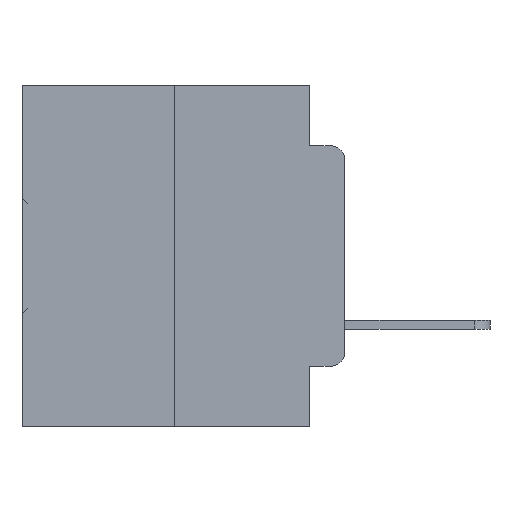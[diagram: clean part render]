
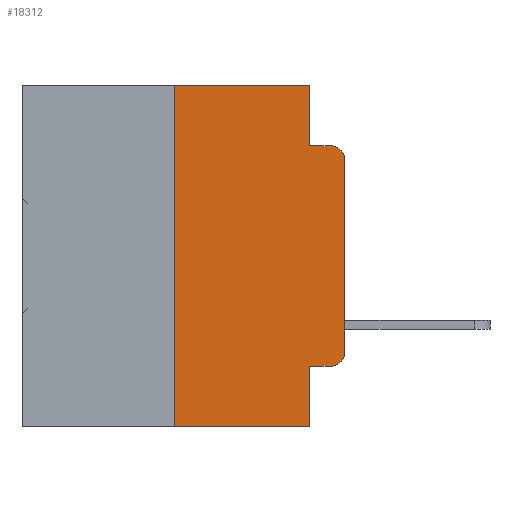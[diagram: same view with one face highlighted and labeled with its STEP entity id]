
A CAD part, left-side view. The second image highlights one B-rep face of the part: STEP entity #18312.
In plain terms, the highlighted planar face has unit normal (-1, 0, 0).
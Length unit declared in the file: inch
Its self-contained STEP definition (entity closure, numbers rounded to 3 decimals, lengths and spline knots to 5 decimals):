
#837 = VECTOR ( 'NONE', #34063, 39.37008 ) ;
#1069 = VERTEX_POINT ( 'NONE', #4931 ) ;
#1289 = DIRECTION ( 'NONE',  ( -1., 0., 0. ) ) ;
#1640 = EDGE_CURVE ( 'NONE', #7655, #21666, #33409, .T. ) ;
#1653 = CARTESIAN_POINT ( 'NONE',  ( 0., 0.051, -0.5 ) ) ;
#2435 = CARTESIAN_POINT ( 'NONE',  ( 0., 0.25, 0. ) ) ;
#2543 = DIRECTION ( 'NONE',  ( 0., 0., -1. ) ) ;
#3406 = VECTOR ( 'NONE', #27637, 39.37008 ) ;
#4751 = CIRCLE ( 'NONE', #5324, 0.02 ) ;
#4931 = CARTESIAN_POINT ( 'NONE',  ( 0., 0., -0.3915 ) ) ;
#5118 = VERTEX_POINT ( 'NONE', #14842 ) ;
#5257 = CARTESIAN_POINT ( 'NONE',  ( 0., 0.25, -0.5 ) ) ;
#5324 = AXIS2_PLACEMENT_3D ( 'NONE', #22847, #22838, #31683 ) ;
#5592 = EDGE_CURVE ( 'NONE', #16302, #21666, #4751, .T. ) ;
#5863 = CARTESIAN_POINT ( 'NONE',  ( 0., 0.473, 0. ) ) ;
#6465 = CARTESIAN_POINT ( 'NONE',  ( 0., 0.473, -0.5 ) ) ;
#6985 = CARTESIAN_POINT ( 'NONE',  ( 0., 0.051, -0.4115 ) ) ;
#7655 = VERTEX_POINT ( 'NONE', #26450 ) ;
#7946 = CARTESIAN_POINT ( 'NONE',  ( 0., 0.02, -0.4115 ) ) ;
#8051 = CIRCLE ( 'NONE', #17934, 0.02 ) ;
#8790 = PLANE ( 'NONE',  #11619 ) ;
#10269 = LINE ( 'NONE', #2435, #22976 ) ;
#10510 = ORIENTED_EDGE ( 'NONE', *, *, #22902, .T. ) ;
#10925 = VECTOR ( 'NONE', #25551, 39.37008 ) ;
#11364 = VERTEX_POINT ( 'NONE', #7946 ) ;
#11619 = AXIS2_PLACEMENT_3D ( 'NONE', #5863, #30052, #14377 ) ;
#11850 = CARTESIAN_POINT ( 'NONE',  ( 0., 0.051, -0.4115 ) ) ;
#12016 = LINE ( 'NONE', #14432, #3406 ) ;
#12131 = ORIENTED_EDGE ( 'NONE', *, *, #5592, .T. ) ;
#12723 = DIRECTION ( 'NONE',  ( 0., -1., 0. ) ) ;
#13222 = EDGE_CURVE ( 'NONE', #1069, #16302, #25636, .T. ) ;
#13951 = CARTESIAN_POINT ( 'NONE',  ( 0., 0.051, 0. ) ) ;
#14268 = CARTESIAN_POINT ( 'NONE',  ( 0., 0.051, -0.0885 ) ) ;
#14276 = DIRECTION ( 'NONE',  ( 0., -1., 0. ) ) ;
#14287 = DIRECTION ( 'NONE',  ( 0., 0., 1. ) ) ;
#14377 = DIRECTION ( 'NONE',  ( 0., 0., -1. ) ) ;
#14432 = CARTESIAN_POINT ( 'NONE',  ( 0., 0.473, 0. ) ) ;
#14842 = CARTESIAN_POINT ( 'NONE',  ( 0., 0.051, 0. ) ) ;
#15081 = ORIENTED_EDGE ( 'NONE', *, *, #13222, .T. ) ;
#15726 = EDGE_CURVE ( 'NONE', #11364, #1069, #8051, .T. ) ;
#16147 = CARTESIAN_POINT ( 'NONE',  ( 0., 0.051, 0. ) ) ;
#16255 = LINE ( 'NONE', #6985, #23364 ) ;
#16302 = VERTEX_POINT ( 'NONE', #28824 ) ;
#17934 = AXIS2_PLACEMENT_3D ( 'NONE', #18211, #1289, #20858 ) ;
#18108 = ORIENTED_EDGE ( 'NONE', *, *, #33627, .F. ) ;
#18178 = LINE ( 'NONE', #6465, #10925 ) ;
#18211 = CARTESIAN_POINT ( 'NONE',  ( 0., 0.02, -0.3915 ) ) ;
#18312 = ADVANCED_FACE ( 'NONE', ( #24898 ), #8790, .F. ) ;
#19654 = EDGE_LOOP ( 'NONE', ( #15081, #12131, #19699, #25568, #18108, #28798, #27617, #25628, #10510, #30363 ) ) ;
#19699 = ORIENTED_EDGE ( 'NONE', *, *, #1640, .F. ) ;
#20858 = DIRECTION ( 'NONE',  ( 0., 0., -1. ) ) ;
#21666 = VERTEX_POINT ( 'NONE', #34697 ) ;
#22262 = LINE ( 'NONE', #16147, #837 ) ;
#22394 = CARTESIAN_POINT ( 'NONE',  ( 0., 0., 0. ) ) ;
#22838 = DIRECTION ( 'NONE',  ( -1., 0., 0. ) ) ;
#22847 = CARTESIAN_POINT ( 'NONE',  ( 0., 0.02, -0.1085 ) ) ;
#22902 = EDGE_CURVE ( 'NONE', #25980, #11364, #16255, .T. ) ;
#22976 = VECTOR ( 'NONE', #24646, 39.37008 ) ;
#23364 = VECTOR ( 'NONE', #12723, 39.37008 ) ;
#23589 = VERTEX_POINT ( 'NONE', #5257 ) ;
#23886 = VECTOR ( 'NONE', #2543, 39.37008 ) ;
#24646 = DIRECTION ( 'NONE',  ( 0., 0., 1. ) ) ;
#24689 = EDGE_CURVE ( 'NONE', #25980, #30252, #22262, .T. ) ;
#24898 = FACE_OUTER_BOUND ( 'NONE', #19654, .T. ) ;
#25551 = DIRECTION ( 'NONE',  ( 0., -1., 0. ) ) ;
#25568 = ORIENTED_EDGE ( 'NONE', *, *, #32974, .F. ) ;
#25628 = ORIENTED_EDGE ( 'NONE', *, *, #24689, .F. ) ;
#25636 = LINE ( 'NONE', #22394, #31478 ) ;
#25980 = VERTEX_POINT ( 'NONE', #11850 ) ;
#26405 = EDGE_CURVE ( 'NONE', #23589, #26705, #10269, .T. ) ;
#26450 = CARTESIAN_POINT ( 'NONE',  ( 0., 0.051, -0.0885 ) ) ;
#26705 = VERTEX_POINT ( 'NONE', #28972 ) ;
#27617 = ORIENTED_EDGE ( 'NONE', *, *, #29566, .T. ) ;
#27637 = DIRECTION ( 'NONE',  ( 0., -1., 0. ) ) ;
#28798 = ORIENTED_EDGE ( 'NONE', *, *, #26405, .F. ) ;
#28824 = CARTESIAN_POINT ( 'NONE',  ( 0., 0., -0.1085 ) ) ;
#28972 = CARTESIAN_POINT ( 'NONE',  ( 0., 0.25, 0. ) ) ;
#29566 = EDGE_CURVE ( 'NONE', #23589, #30252, #18178, .T. ) ;
#30052 = DIRECTION ( 'NONE',  ( 1., 0., 0. ) ) ;
#30252 = VERTEX_POINT ( 'NONE', #1653 ) ;
#30363 = ORIENTED_EDGE ( 'NONE', *, *, #15726, .T. ) ;
#30587 = LINE ( 'NONE', #13951, #23886 ) ;
#31478 = VECTOR ( 'NONE', #14287, 39.37008 ) ;
#31683 = DIRECTION ( 'NONE',  ( 0., 0., -1. ) ) ;
#32974 = EDGE_CURVE ( 'NONE', #5118, #7655, #30587, .T. ) ;
#33409 = LINE ( 'NONE', #14268, #34163 ) ;
#33627 = EDGE_CURVE ( 'NONE', #26705, #5118, #12016, .T. ) ;
#34063 = DIRECTION ( 'NONE',  ( 0., 0., -1. ) ) ;
#34163 = VECTOR ( 'NONE', #14276, 39.37008 ) ;
#34697 = CARTESIAN_POINT ( 'NONE',  ( 0., 0.02, -0.0885 ) ) ;
